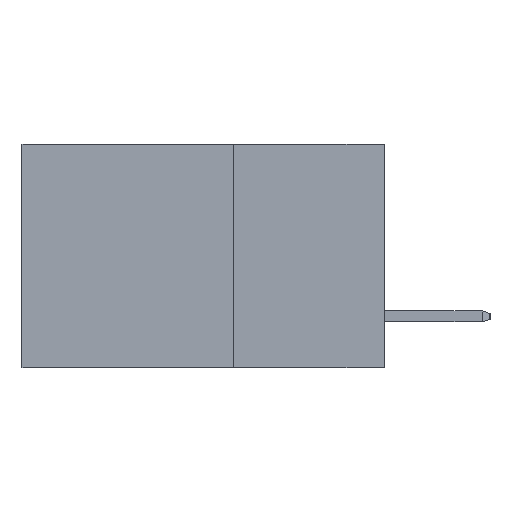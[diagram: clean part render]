
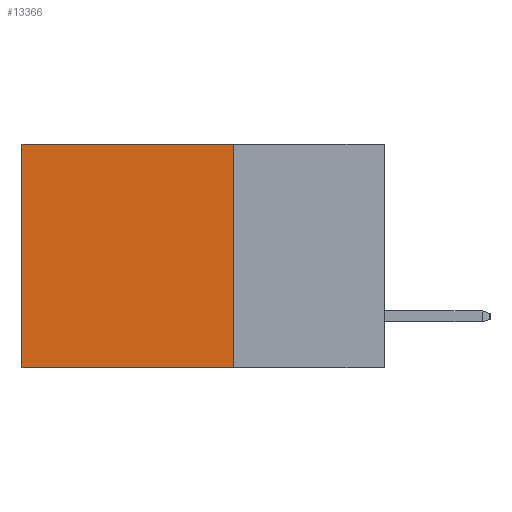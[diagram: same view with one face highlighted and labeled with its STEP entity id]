
A CAD part, left-side view. The second image highlights one B-rep face of the part: STEP entity #13366.
In plain terms, the highlighted planar face has unit normal (-1, 0, 0).
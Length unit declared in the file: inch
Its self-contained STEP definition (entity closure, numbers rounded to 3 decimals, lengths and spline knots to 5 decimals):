
#12 = VECTOR ( 'NONE', #14461, 39.37008 ) ;
#669 = FACE_OUTER_BOUND ( 'NONE', #8749, .T. ) ;
#922 = PLANE ( 'NONE',  #10814 ) ;
#2259 = CARTESIAN_POINT ( 'NONE',  ( 0.298, 0.25, -0.37 ) ) ;
#2712 = DIRECTION ( 'NONE',  ( 0., 0., -1. ) ) ;
#3288 = LINE ( 'NONE', #15400, #15641 ) ;
#3311 = LINE ( 'NONE', #2259, #12716 ) ;
#3585 = DIRECTION ( 'NONE',  ( 1., 0., 0. ) ) ;
#4848 = EDGE_CURVE ( 'NONE', #15374, #9571, #3311, .T. ) ;
#5910 = VECTOR ( 'NONE', #2712, 39.37008 ) ;
#6295 = LINE ( 'NONE', #12517, #5910 ) ;
#6309 = EDGE_CURVE ( 'NONE', #7787, #15374, #3288, .T. ) ;
#6502 = CARTESIAN_POINT ( 'NONE',  ( 0.298, 0.6, -0.37 ) ) ;
#6975 = LINE ( 'NONE', #7343, #12 ) ;
#7217 = EDGE_CURVE ( 'NONE', #11737, #9571, #6295, .T. ) ;
#7271 = CARTESIAN_POINT ( 'NONE',  ( 0.298, 0.25, 0. ) ) ;
#7343 = CARTESIAN_POINT ( 'NONE',  ( 0.298, 0.25, 0. ) ) ;
#7787 = VERTEX_POINT ( 'NONE', #11339 ) ;
#8749 = EDGE_LOOP ( 'NONE', ( #14326, #14299, #14273, #13964 ) ) ;
#8910 = DIRECTION ( 'NONE',  ( 0., 1., 0. ) ) ;
#9353 = EDGE_CURVE ( 'NONE', #7787, #11737, #6975, .T. ) ;
#9545 = CARTESIAN_POINT ( 'NONE',  ( 0.298, 0.25, -0.37 ) ) ;
#9571 = VERTEX_POINT ( 'NONE', #6502 ) ;
#10814 = AXIS2_PLACEMENT_3D ( 'NONE', #7271, #3585, #12172 ) ;
#10828 = DIRECTION ( 'NONE',  ( 0., 0., -1. ) ) ;
#11339 = CARTESIAN_POINT ( 'NONE',  ( 0.298, 0.25, 0. ) ) ;
#11737 = VERTEX_POINT ( 'NONE', #15071 ) ;
#12172 = DIRECTION ( 'NONE',  ( 0., 0., -1. ) ) ;
#12517 = CARTESIAN_POINT ( 'NONE',  ( 0.298, 0.6, 0. ) ) ;
#12716 = VECTOR ( 'NONE', #8910, 39.37008 ) ;
#13366 = ADVANCED_FACE ( 'NONE', ( #669 ), #922, .F. ) ;
#13964 = ORIENTED_EDGE ( 'NONE', *, *, #9353, .T. ) ;
#14273 = ORIENTED_EDGE ( 'NONE', *, *, #6309, .F. ) ;
#14299 = ORIENTED_EDGE ( 'NONE', *, *, #4848, .F. ) ;
#14326 = ORIENTED_EDGE ( 'NONE', *, *, #7217, .T. ) ;
#14461 = DIRECTION ( 'NONE',  ( 0., 1., 0. ) ) ;
#15071 = CARTESIAN_POINT ( 'NONE',  ( 0.298, 0.6, 0. ) ) ;
#15374 = VERTEX_POINT ( 'NONE', #9545 ) ;
#15400 = CARTESIAN_POINT ( 'NONE',  ( 0.298, 0.25, 0. ) ) ;
#15641 = VECTOR ( 'NONE', #10828, 39.37008 ) ;
